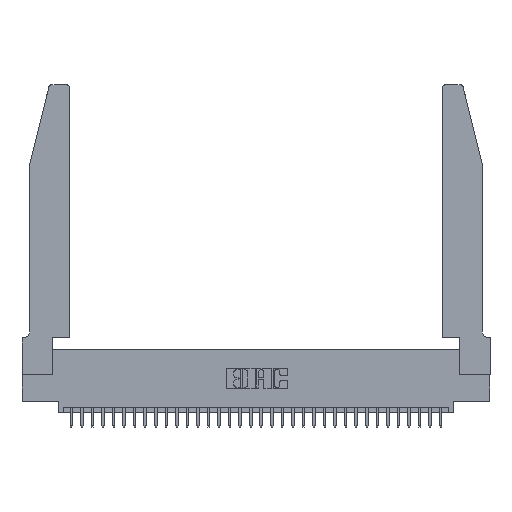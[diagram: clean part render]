
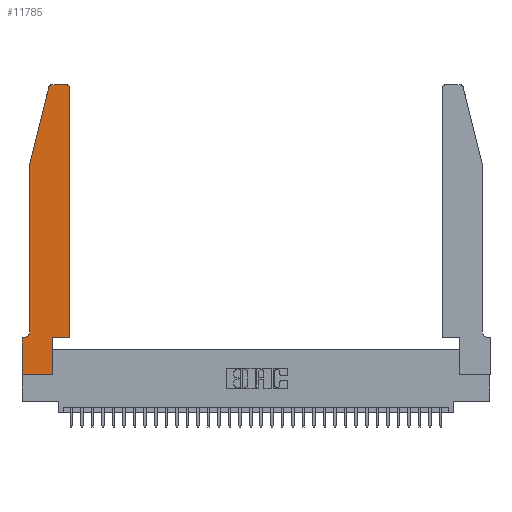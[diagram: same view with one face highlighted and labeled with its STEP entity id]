
A CAD part, top view. The second image highlights one B-rep face of the part: STEP entity #11785.
In plain terms, the highlighted planar face has unit normal (0, 0, 1).
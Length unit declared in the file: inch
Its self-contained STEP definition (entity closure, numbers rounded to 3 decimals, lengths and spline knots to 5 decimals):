
#305 = CARTESIAN_POINT ( 'NONE',  ( 0.0055, 0.35, 0.37 ) ) ;
#537 = CARTESIAN_POINT ( 'NONE',  ( 0., 0.35, 0.37 ) ) ;
#1952 = EDGE_CURVE ( 'NONE', #7930, #19045, #28091, .T. ) ;
#2008 = CARTESIAN_POINT ( 'NONE',  ( 0.2865, 0., 0.37 ) ) ;
#2346 = DIRECTION ( 'NONE',  ( 1., 0., 0. ) ) ;
#3107 = EDGE_CURVE ( 'NONE', #6613, #4905, #16139, .T. ) ;
#3225 = PLANE ( 'NONE',  #9766 ) ;
#3347 = DIRECTION ( 'NONE',  ( -1., 0., 0. ) ) ;
#4323 = VERTEX_POINT ( 'NONE', #28085 ) ;
#4565 = ORIENTED_EDGE ( 'NONE', *, *, #15061, .T. ) ;
#4681 = LINE ( 'NONE', #28929, #17857 ) ;
#4816 = VECTOR ( 'NONE', #21720, 39.37008 ) ;
#4905 = VERTEX_POINT ( 'NONE', #2008 ) ;
#5264 = ORIENTED_EDGE ( 'NONE', *, *, #6820, .T. ) ;
#5269 = VERTEX_POINT ( 'NONE', #26155 ) ;
#5510 = DIRECTION ( 'NONE',  ( 1., 0., 0. ) ) ;
#5674 = CARTESIAN_POINT ( 'NONE',  ( 0.2865, 0.35, 0.37 ) ) ;
#6229 = CARTESIAN_POINT ( 'NONE',  ( 0.284, 2.72, 0.37 ) ) ;
#6328 = VECTOR ( 'NONE', #5510, 39.37008 ) ;
#6613 = VERTEX_POINT ( 'NONE', #19168 ) ;
#6757 = DIRECTION ( 'NONE',  ( -0.239, -0.971, 0. ) ) ;
#6820 = EDGE_CURVE ( 'NONE', #19710, #4323, #10998, .T. ) ;
#7285 = EDGE_CURVE ( 'NONE', #5269, #30782, #30214, .T. ) ;
#7417 = VECTOR ( 'NONE', #11445, 39.37008 ) ;
#7633 = VERTEX_POINT ( 'NONE', #12571 ) ;
#7699 = CARTESIAN_POINT ( 'NONE',  ( 0.25487, 2.72718, 0.37 ) ) ;
#7930 = VERTEX_POINT ( 'NONE', #5674 ) ;
#8463 = ORIENTED_EDGE ( 'NONE', *, *, #8472, .T. ) ;
#8472 = EDGE_CURVE ( 'NONE', #19045, #7633, #4681, .T. ) ;
#8521 = DIRECTION ( 'NONE',  ( 1., 0., 0. ) ) ;
#8695 = CARTESIAN_POINT ( 'NONE',  ( 0.0055, 0.42, 0.37 ) ) ;
#8888 = DIRECTION ( 'NONE',  ( 1., 0., 0. ) ) ;
#9766 = AXIS2_PLACEMENT_3D ( 'NONE', #537, #24227, #8521 ) ;
#10736 = ORIENTED_EDGE ( 'NONE', *, *, #19233, .T. ) ;
#10998 = LINE ( 'NONE', #25105, #17186 ) ;
#11101 = FACE_OUTER_BOUND ( 'NONE', #31992, .T. ) ;
#11163 = AXIS2_PLACEMENT_3D ( 'NONE', #14301, #32595, #16945 ) ;
#11276 = CARTESIAN_POINT ( 'NONE',  ( 0.0755, 0.35, 0.37 ) ) ;
#11331 = DIRECTION ( 'NONE',  ( -1., 0., 0. ) ) ;
#11445 = DIRECTION ( 'NONE',  ( 0., -1., 0. ) ) ;
#11608 = ORIENTED_EDGE ( 'NONE', *, *, #16807, .T. ) ;
#11785 = ADVANCED_FACE ( 'NONE', ( #11101 ), #3225, .T. ) ;
#12571 = CARTESIAN_POINT ( 'NONE',  ( 0.4505, 2.72, 0.37 ) ) ;
#12845 = DIRECTION ( 'NONE',  ( 0., -1., 0. ) ) ;
#14059 = EDGE_CURVE ( 'NONE', #4905, #7930, #14468, .T. ) ;
#14301 = CARTESIAN_POINT ( 'NONE',  ( 0.4205, 2.72, 0.37 ) ) ;
#14468 = LINE ( 'NONE', #15552, #28405 ) ;
#15061 = EDGE_CURVE ( 'NONE', #4323, #5269, #15251, .T. ) ;
#15251 = LINE ( 'NONE', #21896, #7417 ) ;
#15285 = CARTESIAN_POINT ( 'NONE',  ( 0., 0.35, 0.37 ) ) ;
#15425 = AXIS2_PLACEMENT_3D ( 'NONE', #8695, #27052, #11331 ) ;
#15552 = CARTESIAN_POINT ( 'NONE',  ( 0.2865, 0.35, 0.37 ) ) ;
#15949 = CIRCLE ( 'NONE', #11163, 0.03 ) ;
#15999 = CARTESIAN_POINT ( 'NONE',  ( 0.4505, 0.35, 0.37 ) ) ;
#16139 = LINE ( 'NONE', #18092, #23101 ) ;
#16597 = VERTEX_POINT ( 'NONE', #15285 ) ;
#16807 = EDGE_CURVE ( 'NONE', #7633, #32696, #15949, .T. ) ;
#16945 = DIRECTION ( 'NONE',  ( 1., 0., 0. ) ) ;
#17186 = VECTOR ( 'NONE', #6757, 39.37008 ) ;
#17857 = VECTOR ( 'NONE', #31547, 39.37008 ) ;
#18066 = ORIENTED_EDGE ( 'NONE', *, *, #3107, .T. ) ;
#18092 = CARTESIAN_POINT ( 'NONE',  ( 0., 0., 0.37 ) ) ;
#18960 = ORIENTED_EDGE ( 'NONE', *, *, #25822, .T. ) ;
#19045 = VERTEX_POINT ( 'NONE', #21022 ) ;
#19083 = CARTESIAN_POINT ( 'NONE',  ( 0.2605, 2.75, 0.37 ) ) ;
#19095 = LINE ( 'NONE', #11276, #25237 ) ;
#19168 = CARTESIAN_POINT ( 'NONE',  ( 0., 0., 0.37 ) ) ;
#19233 = EDGE_CURVE ( 'NONE', #30782, #16597, #19095, .T. ) ;
#19710 = VERTEX_POINT ( 'NONE', #7699 ) ;
#21022 = CARTESIAN_POINT ( 'NONE',  ( 0.4505, 0.35, 0.37 ) ) ;
#21350 = VERTEX_POINT ( 'NONE', #23694 ) ;
#21610 = ORIENTED_EDGE ( 'NONE', *, *, #14059, .T. ) ;
#21720 = DIRECTION ( 'NONE',  ( -1., 0., 0. ) ) ;
#21896 = CARTESIAN_POINT ( 'NONE',  ( 0.0755, 2., 0.37 ) ) ;
#23101 = VECTOR ( 'NONE', #2346, 39.37008 ) ;
#23694 = CARTESIAN_POINT ( 'NONE',  ( 0.284, 2.75, 0.37 ) ) ;
#24227 = DIRECTION ( 'NONE',  ( 0., 0., 1. ) ) ;
#24586 = DIRECTION ( 'NONE',  ( 0., 0., 1. ) ) ;
#24806 = EDGE_CURVE ( 'NONE', #32696, #21350, #25786, .T. ) ;
#24937 = ORIENTED_EDGE ( 'NONE', *, *, #1952, .T. ) ;
#25105 = CARTESIAN_POINT ( 'NONE',  ( 0.0755, 2., 0.37 ) ) ;
#25237 = VECTOR ( 'NONE', #3347, 39.37008 ) ;
#25279 = VECTOR ( 'NONE', #12845, 39.37008 ) ;
#25786 = LINE ( 'NONE', #19083, #4816 ) ;
#25822 = EDGE_CURVE ( 'NONE', #16597, #6613, #33038, .T. ) ;
#26155 = CARTESIAN_POINT ( 'NONE',  ( 0.0755, 0.42, 0.37 ) ) ;
#27052 = DIRECTION ( 'NONE',  ( 0., 0., -1. ) ) ;
#28085 = CARTESIAN_POINT ( 'NONE',  ( 0.0755, 2., 0.37 ) ) ;
#28091 = LINE ( 'NONE', #15999, #6328 ) ;
#28405 = VECTOR ( 'NONE', #33815, 39.37008 ) ;
#28570 = CARTESIAN_POINT ( 'NONE',  ( 0., 0., 0.37 ) ) ;
#28654 = ORIENTED_EDGE ( 'NONE', *, *, #31812, .T. ) ;
#28792 = CIRCLE ( 'NONE', #28920, 0.03 ) ;
#28920 = AXIS2_PLACEMENT_3D ( 'NONE', #6229, #24586, #8888 ) ;
#28929 = CARTESIAN_POINT ( 'NONE',  ( 0.4505, 0.35, 0.37 ) ) ;
#29640 = ORIENTED_EDGE ( 'NONE', *, *, #24806, .T. ) ;
#30214 = CIRCLE ( 'NONE', #15425, 0.07 ) ;
#30691 = CARTESIAN_POINT ( 'NONE',  ( 0.4205, 2.75, 0.37 ) ) ;
#30782 = VERTEX_POINT ( 'NONE', #305 ) ;
#31547 = DIRECTION ( 'NONE',  ( 0., 1., 0. ) ) ;
#31812 = EDGE_CURVE ( 'NONE', #21350, #19710, #28792, .T. ) ;
#31992 = EDGE_LOOP ( 'NONE', ( #29640, #28654, #5264, #4565, #33796, #10736, #18960, #18066, #21610, #24937, #8463, #11608 ) ) ;
#32595 = DIRECTION ( 'NONE',  ( 0., 0., 1. ) ) ;
#32696 = VERTEX_POINT ( 'NONE', #30691 ) ;
#33038 = LINE ( 'NONE', #28570, #25279 ) ;
#33796 = ORIENTED_EDGE ( 'NONE', *, *, #7285, .T. ) ;
#33815 = DIRECTION ( 'NONE',  ( 0., 1., 0. ) ) ;
